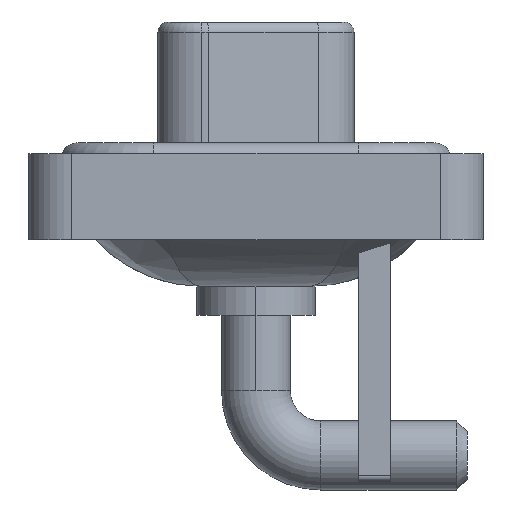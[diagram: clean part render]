
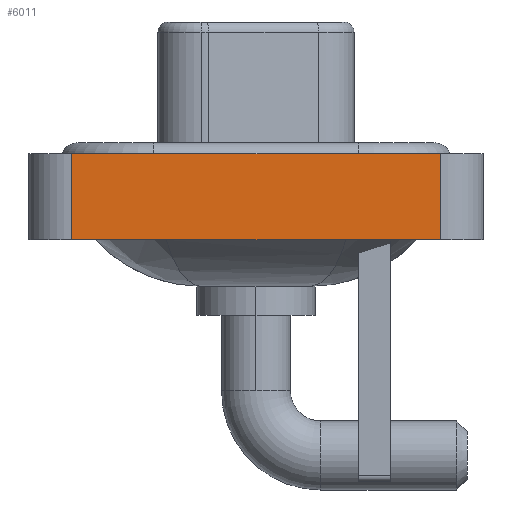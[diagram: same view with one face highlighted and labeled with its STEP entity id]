
A CAD part, left-side view. The second image highlights one B-rep face of the part: STEP entity #6011.
In plain terms, the highlighted planar face has unit normal (-1, 0, 0).
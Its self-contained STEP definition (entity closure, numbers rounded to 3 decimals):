
#70 = EDGE_LOOP ( 'NONE', ( #1954, #121, #1606, #7867 ) ) ;
#121 = ORIENTED_EDGE ( 'NONE', *, *, #13197, .F. ) ;
#614 = DIRECTION ( 'NONE',  ( 0., 0., 1. ) ) ;
#821 = CARTESIAN_POINT ( 'NONE',  ( -7.25, -8.55, -3.6 ) ) ;
#984 = DIRECTION ( 'NONE',  ( 0., -1., 0. ) ) ;
#1606 = ORIENTED_EDGE ( 'NONE', *, *, #11014, .F. ) ;
#1666 = FACE_OUTER_BOUND ( 'NONE', #70, .T. ) ;
#1864 = DIRECTION ( 'NONE',  ( 0., 0., 1. ) ) ;
#1917 = EDGE_CURVE ( 'NONE', #10168, #12653, #6593, .T. ) ;
#1954 = ORIENTED_EDGE ( 'NONE', *, *, #1917, .T. ) ;
#2023 = LINE ( 'NONE', #821, #9208 ) ;
#2650 = CARTESIAN_POINT ( 'NONE',  ( -7.25, 8.55, -3.6 ) ) ;
#4134 = DIRECTION ( 'NONE',  ( 0., 0., 1. ) ) ;
#4525 = AXIS2_PLACEMENT_3D ( 'NONE', #10246, #11604, #614 ) ;
#4834 = DIRECTION ( 'NONE',  ( 0., -1., 0. ) ) ;
#5347 = PLANE ( 'NONE',  #4525 ) ;
#6011 = ADVANCED_FACE ( 'NONE', ( #1666 ), #5347, .T. ) ;
#6593 = LINE ( 'NONE', #12766, #8928 ) ;
#7036 = EDGE_CURVE ( 'NONE', #13652, #10168, #2023, .T. ) ;
#7867 = ORIENTED_EDGE ( 'NONE', *, *, #7036, .T. ) ;
#8928 = VECTOR ( 'NONE', #1864, 1000. ) ;
#9015 = VECTOR ( 'NONE', #4834, 1000. ) ;
#9208 = VECTOR ( 'NONE', #984, 1000. ) ;
#9716 = CARTESIAN_POINT ( 'NONE',  ( -7.25, -8.55, -3.6 ) ) ;
#10069 = CARTESIAN_POINT ( 'NONE',  ( -7.25, -8.55, 0.4 ) ) ;
#10168 = VERTEX_POINT ( 'NONE', #9716 ) ;
#10235 = LINE ( 'NONE', #15104, #13106 ) ;
#10246 = CARTESIAN_POINT ( 'NONE',  ( -7.25, -8.55, -3.6 ) ) ;
#11014 = EDGE_CURVE ( 'NONE', #13652, #12731, #10235, .T. ) ;
#11604 = DIRECTION ( 'NONE',  ( -1., 0., 0. ) ) ;
#12653 = VERTEX_POINT ( 'NONE', #10069 ) ;
#12731 = VERTEX_POINT ( 'NONE', #15082 ) ;
#12766 = CARTESIAN_POINT ( 'NONE',  ( -7.25, -8.55, -3.6 ) ) ;
#13106 = VECTOR ( 'NONE', #4134, 1000. ) ;
#13197 = EDGE_CURVE ( 'NONE', #12731, #12653, #14757, .T. ) ;
#13652 = VERTEX_POINT ( 'NONE', #2650 ) ;
#14757 = LINE ( 'NONE', #15800, #9015 ) ;
#15082 = CARTESIAN_POINT ( 'NONE',  ( -7.25, 8.55, 0.4 ) ) ;
#15104 = CARTESIAN_POINT ( 'NONE',  ( -7.25, 8.55, -3.6 ) ) ;
#15800 = CARTESIAN_POINT ( 'NONE',  ( -7.25, -8.55, 0.4 ) ) ;
